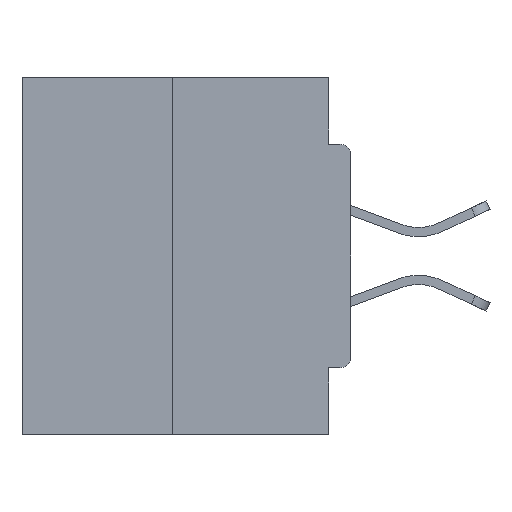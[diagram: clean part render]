
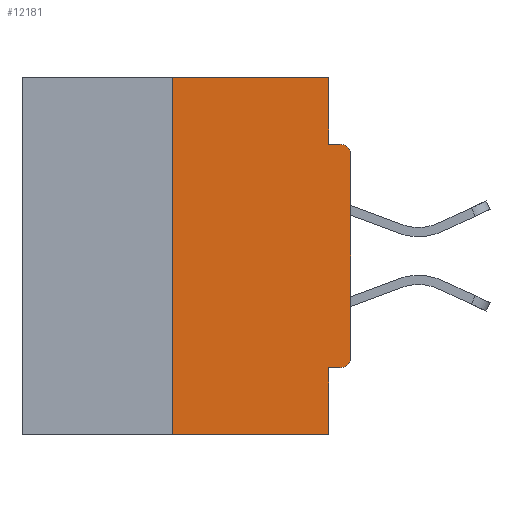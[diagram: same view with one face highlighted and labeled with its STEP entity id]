
A CAD part, left-side view. The second image highlights one B-rep face of the part: STEP entity #12181.
In plain terms, the highlighted planar face has unit normal (-1, 0, 0).
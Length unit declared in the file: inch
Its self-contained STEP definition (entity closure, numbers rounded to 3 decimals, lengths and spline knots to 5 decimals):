
#131 = DIRECTION ( 'NONE',  ( 0., 1., 0. ) ) ;
#615 = VECTOR ( 'NONE', #13128, 39.37008 ) ;
#639 = CARTESIAN_POINT ( 'NONE',  ( 0., 0.031, -0.0935 ) ) ;
#1458 = DIRECTION ( 'NONE',  ( 0., -1., 0. ) ) ;
#1502 = CARTESIAN_POINT ( 'NONE',  ( 0., 0.46, 0. ) ) ;
#1708 = VECTOR ( 'NONE', #1458, 39.37008 ) ;
#3023 = CARTESIAN_POINT ( 'NONE',  ( 0., 0.031, 0. ) ) ;
#3295 = DIRECTION ( 'NONE',  ( 0., 0., 1. ) ) ;
#3327 = AXIS2_PLACEMENT_3D ( 'NONE', #27205, #21031, #21780 ) ;
#4259 = CARTESIAN_POINT ( 'NONE',  ( 0., 0.46, 0. ) ) ;
#4446 = PLANE ( 'NONE',  #14488 ) ;
#4574 = DIRECTION ( 'NONE',  ( 0., 0., -1. ) ) ;
#4634 = AXIS2_PLACEMENT_3D ( 'NONE', #23705, #26557, #9734 ) ;
#4728 = VECTOR ( 'NONE', #25734, 39.37008 ) ;
#4762 = VERTEX_POINT ( 'NONE', #3023 ) ;
#5197 = VECTOR ( 'NONE', #7093, 39.37008 ) ;
#5799 = EDGE_CURVE ( 'NONE', #29366, #22229, #6967, .T. ) ;
#5920 = LINE ( 'NONE', #10622, #615 ) ;
#6021 = EDGE_CURVE ( 'NONE', #11073, #4762, #25836, .T. ) ;
#6284 = LINE ( 'NONE', #22248, #12403 ) ;
#6835 = VERTEX_POINT ( 'NONE', #14175 ) ;
#6937 = CARTESIAN_POINT ( 'NONE',  ( 0., 0.031, -0.5 ) ) ;
#6967 = LINE ( 'NONE', #14201, #28435 ) ;
#6988 = ORIENTED_EDGE ( 'NONE', *, *, #35061, .F. ) ;
#6999 = CIRCLE ( 'NONE', #4634, 0.015 ) ;
#7093 = DIRECTION ( 'NONE',  ( 0., -1., 0. ) ) ;
#7150 = CARTESIAN_POINT ( 'NONE',  ( 0., 0.031, -0.4065 ) ) ;
#7863 = LINE ( 'NONE', #9684, #1708 ) ;
#8153 = ORIENTED_EDGE ( 'NONE', *, *, #6021, .F. ) ;
#8913 = EDGE_CURVE ( 'NONE', #15291, #24432, #5920, .T. ) ;
#9684 = CARTESIAN_POINT ( 'NONE',  ( 0., 0.46, -0.5 ) ) ;
#9734 = DIRECTION ( 'NONE',  ( 0., 0., -1. ) ) ;
#10072 = DIRECTION ( 'NONE',  ( 1., 0., 0. ) ) ;
#10622 = CARTESIAN_POINT ( 'NONE',  ( 0., 0.031, -0.5 ) ) ;
#11073 = VERTEX_POINT ( 'NONE', #28049 ) ;
#11773 = LINE ( 'NONE', #25936, #27131 ) ;
#12181 = ADVANCED_FACE ( 'NONE', ( #14115 ), #4446, .F. ) ;
#12251 = CARTESIAN_POINT ( 'NONE',  ( 0., 0., -0.1085 ) ) ;
#12273 = DIRECTION ( 'NONE',  ( 0., 0., 1. ) ) ;
#12403 = VECTOR ( 'NONE', #24983, 39.37008 ) ;
#13128 = DIRECTION ( 'NONE',  ( 0., 0., -1. ) ) ;
#14115 = FACE_OUTER_BOUND ( 'NONE', #33554, .T. ) ;
#14175 = CARTESIAN_POINT ( 'NONE',  ( 0., 0.015, -0.0935 ) ) ;
#14201 = CARTESIAN_POINT ( 'NONE',  ( 0., 0., 0. ) ) ;
#14488 = AXIS2_PLACEMENT_3D ( 'NONE', #1502, #10072, #4574 ) ;
#14740 = CARTESIAN_POINT ( 'NONE',  ( 0., 0., -0.3915 ) ) ;
#15212 = LINE ( 'NONE', #16572, #4728 ) ;
#15291 = VERTEX_POINT ( 'NONE', #7150 ) ;
#15585 = EDGE_CURVE ( 'NONE', #30890, #15291, #32394, .T. ) ;
#15804 = EDGE_CURVE ( 'NONE', #22229, #6835, #18762, .T. ) ;
#16176 = ORIENTED_EDGE ( 'NONE', *, *, #20682, .T. ) ;
#16572 = CARTESIAN_POINT ( 'NONE',  ( 0., 0., -0.0935 ) ) ;
#17839 = ORIENTED_EDGE ( 'NONE', *, *, #15585, .F. ) ;
#18329 = VECTOR ( 'NONE', #131, 39.37008 ) ;
#18762 = CIRCLE ( 'NONE', #3327, 0.015 ) ;
#20682 = EDGE_CURVE ( 'NONE', #30890, #29366, #6999, .T. ) ;
#20748 = ORIENTED_EDGE ( 'NONE', *, *, #8913, .F. ) ;
#21031 = DIRECTION ( 'NONE',  ( -1., 0., 0. ) ) ;
#21780 = DIRECTION ( 'NONE',  ( 0., 0., -1. ) ) ;
#22164 = VERTEX_POINT ( 'NONE', #639 ) ;
#22229 = VERTEX_POINT ( 'NONE', #12251 ) ;
#22248 = CARTESIAN_POINT ( 'NONE',  ( 0., 0.031, 0. ) ) ;
#23705 = CARTESIAN_POINT ( 'NONE',  ( 0., 0.015, -0.3915 ) ) ;
#24082 = EDGE_CURVE ( 'NONE', #22164, #6835, #15212, .T. ) ;
#24432 = VERTEX_POINT ( 'NONE', #6937 ) ;
#24983 = DIRECTION ( 'NONE',  ( 0., 0., -1. ) ) ;
#25543 = CARTESIAN_POINT ( 'NONE',  ( 0., 0., -0.4065 ) ) ;
#25566 = CARTESIAN_POINT ( 'NONE',  ( 0., 0.015, -0.4065 ) ) ;
#25734 = DIRECTION ( 'NONE',  ( 0., -1., 0. ) ) ;
#25836 = LINE ( 'NONE', #4259, #5197 ) ;
#25936 = CARTESIAN_POINT ( 'NONE',  ( 0., 0.25, 0. ) ) ;
#26557 = DIRECTION ( 'NONE',  ( -1., 0., 0. ) ) ;
#27131 = VECTOR ( 'NONE', #12273, 39.37008 ) ;
#27205 = CARTESIAN_POINT ( 'NONE',  ( 0., 0.015, -0.1085 ) ) ;
#27647 = ORIENTED_EDGE ( 'NONE', *, *, #33189, .T. ) ;
#28049 = CARTESIAN_POINT ( 'NONE',  ( 0., 0.25, 0. ) ) ;
#28435 = VECTOR ( 'NONE', #3295, 39.37008 ) ;
#29012 = VERTEX_POINT ( 'NONE', #34315 ) ;
#29366 = VERTEX_POINT ( 'NONE', #14740 ) ;
#29592 = ORIENTED_EDGE ( 'NONE', *, *, #15804, .T. ) ;
#30869 = ORIENTED_EDGE ( 'NONE', *, *, #34156, .F. ) ;
#30890 = VERTEX_POINT ( 'NONE', #25566 ) ;
#32394 = LINE ( 'NONE', #25543, #18329 ) ;
#32591 = ORIENTED_EDGE ( 'NONE', *, *, #5799, .T. ) ;
#33189 = EDGE_CURVE ( 'NONE', #29012, #24432, #7863, .T. ) ;
#33554 = EDGE_LOOP ( 'NONE', ( #8153, #30869, #27647, #20748, #17839, #16176, #32591, #29592, #34747, #6988 ) ) ;
#34156 = EDGE_CURVE ( 'NONE', #29012, #11073, #11773, .T. ) ;
#34315 = CARTESIAN_POINT ( 'NONE',  ( 0., 0.25, -0.5 ) ) ;
#34747 = ORIENTED_EDGE ( 'NONE', *, *, #24082, .F. ) ;
#35061 = EDGE_CURVE ( 'NONE', #4762, #22164, #6284, .T. ) ;
